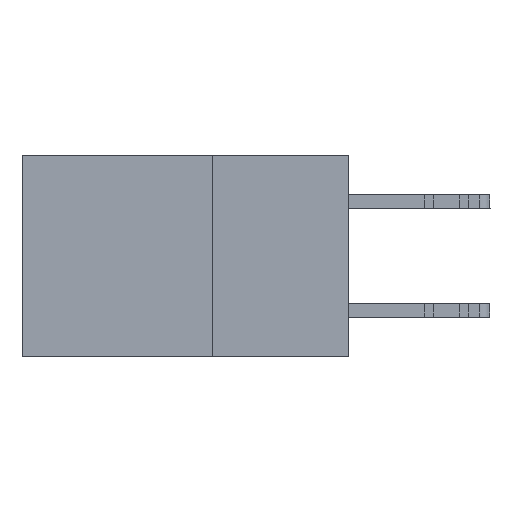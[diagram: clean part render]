
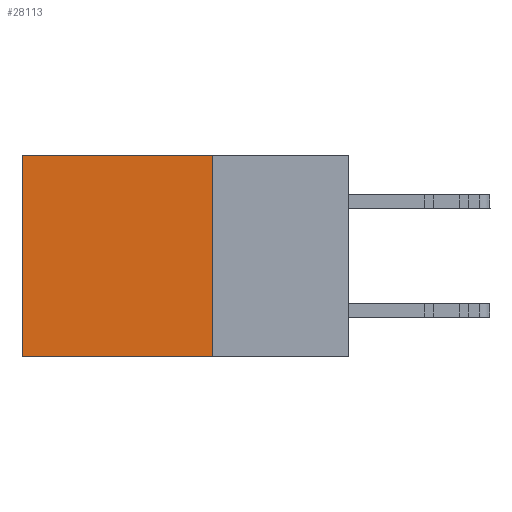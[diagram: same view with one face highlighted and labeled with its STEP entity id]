
A CAD part, left-side view. The second image highlights one B-rep face of the part: STEP entity #28113.
In plain terms, the highlighted planar face has unit normal (-1, 0, 0).
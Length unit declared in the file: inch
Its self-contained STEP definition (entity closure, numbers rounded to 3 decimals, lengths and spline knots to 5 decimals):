
#111 = EDGE_LOOP ( 'NONE', ( #7778, #25163, #28363, #19896 ) ) ;
#152 = EDGE_CURVE ( 'NONE', #25813, #12421, #12470, .T. ) ;
#1504 = DIRECTION ( 'NONE',  ( 0., 0., -1. ) ) ;
#1709 = PLANE ( 'NONE',  #22006 ) ;
#1862 = FACE_OUTER_BOUND ( 'NONE', #111, .T. ) ;
#2232 = LINE ( 'NONE', #9450, #26491 ) ;
#2956 = CARTESIAN_POINT ( 'NONE',  ( 0.298, 0.6, 0. ) ) ;
#4306 = CARTESIAN_POINT ( 'NONE',  ( 0.298, 0.25, 0. ) ) ;
#6829 = EDGE_CURVE ( 'NONE', #13004, #17055, #7258, .T. ) ;
#7258 = LINE ( 'NONE', #18071, #29576 ) ;
#7778 = ORIENTED_EDGE ( 'NONE', *, *, #30641, .T. ) ;
#8196 = DIRECTION ( 'NONE',  ( 0., 0., -1. ) ) ;
#9450 = CARTESIAN_POINT ( 'NONE',  ( 0.298, 0.25, 0. ) ) ;
#12421 = VERTEX_POINT ( 'NONE', #32387 ) ;
#12470 = LINE ( 'NONE', #31533, #13631 ) ;
#13004 = VERTEX_POINT ( 'NONE', #31364 ) ;
#13202 = LINE ( 'NONE', #2956, #20618 ) ;
#13631 = VECTOR ( 'NONE', #13916, 39.37008 ) ;
#13916 = DIRECTION ( 'NONE',  ( 0., 1., 0. ) ) ;
#14507 = CARTESIAN_POINT ( 'NONE',  ( 0.298, 0.6, 0. ) ) ;
#17055 = VERTEX_POINT ( 'NONE', #14507 ) ;
#18071 = CARTESIAN_POINT ( 'NONE',  ( 0.298, 0.25, 0. ) ) ;
#18289 = DIRECTION ( 'NONE',  ( 0., 1., 0. ) ) ;
#18643 = CARTESIAN_POINT ( 'NONE',  ( 0.298, 0.25, -0.37 ) ) ;
#19168 = DIRECTION ( 'NONE',  ( 1., 0., 0. ) ) ;
#19896 = ORIENTED_EDGE ( 'NONE', *, *, #6829, .T. ) ;
#20618 = VECTOR ( 'NONE', #8196, 39.37008 ) ;
#22006 = AXIS2_PLACEMENT_3D ( 'NONE', #4306, #19168, #29270 ) ;
#25163 = ORIENTED_EDGE ( 'NONE', *, *, #152, .F. ) ;
#25813 = VERTEX_POINT ( 'NONE', #18643 ) ;
#26491 = VECTOR ( 'NONE', #1504, 39.37008 ) ;
#28113 = ADVANCED_FACE ( 'NONE', ( #1862 ), #1709, .F. ) ;
#28234 = EDGE_CURVE ( 'NONE', #13004, #25813, #2232, .T. ) ;
#28363 = ORIENTED_EDGE ( 'NONE', *, *, #28234, .F. ) ;
#29270 = DIRECTION ( 'NONE',  ( 0., 0., -1. ) ) ;
#29576 = VECTOR ( 'NONE', #18289, 39.37008 ) ;
#30641 = EDGE_CURVE ( 'NONE', #17055, #12421, #13202, .T. ) ;
#31364 = CARTESIAN_POINT ( 'NONE',  ( 0.298, 0.25, 0. ) ) ;
#31533 = CARTESIAN_POINT ( 'NONE',  ( 0.298, 0.25, -0.37 ) ) ;
#32387 = CARTESIAN_POINT ( 'NONE',  ( 0.298, 0.6, -0.37 ) ) ;
